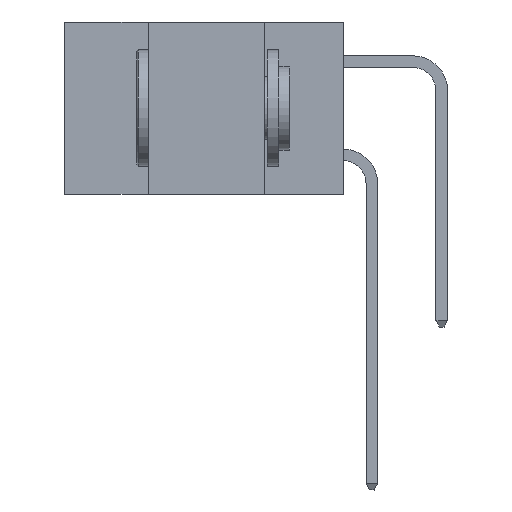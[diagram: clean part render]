
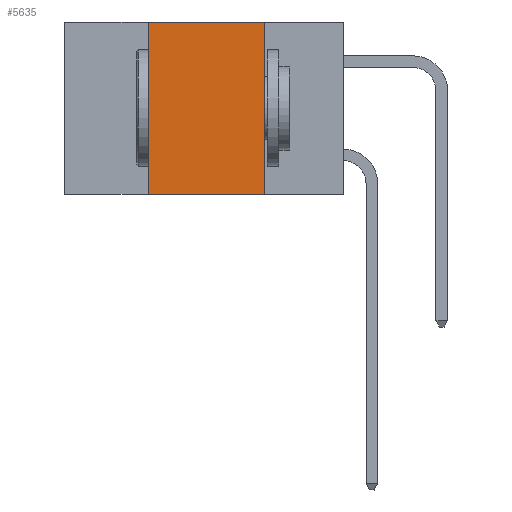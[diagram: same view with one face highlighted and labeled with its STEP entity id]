
A CAD part, left-side view. The second image highlights one B-rep face of the part: STEP entity #5635.
In plain terms, the highlighted planar face has unit normal (-1, 0, 0).
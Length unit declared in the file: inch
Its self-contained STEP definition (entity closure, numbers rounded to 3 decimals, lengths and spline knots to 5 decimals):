
#769 = CARTESIAN_POINT ( 'NONE',  ( 0., 0.17, 0. ) ) ;
#1058 = LINE ( 'NONE', #2823, #28242 ) ;
#1062 = EDGE_CURVE ( 'NONE', #29601, #11654, #19205, .T. ) ;
#1976 = CARTESIAN_POINT ( 'NONE',  ( 0., 0.6, -0.37 ) ) ;
#2430 = EDGE_LOOP ( 'NONE', ( #25160, #31575, #11569, #6998 ) ) ;
#2725 = CARTESIAN_POINT ( 'NONE',  ( 0., 0.6, 0. ) ) ;
#2823 = CARTESIAN_POINT ( 'NONE',  ( 0., 0.42, 0. ) ) ;
#3023 = CARTESIAN_POINT ( 'NONE',  ( 0., 0.6, 0. ) ) ;
#3676 = CARTESIAN_POINT ( 'NONE',  ( 0., 0.42, 0. ) ) ;
#4489 = VECTOR ( 'NONE', #7281, 39.37008 ) ;
#5635 = ADVANCED_FACE ( 'NONE', ( #14185 ), #13367, .F. ) ;
#6341 = EDGE_CURVE ( 'NONE', #23359, #29601, #26075, .T. ) ;
#6998 = ORIENTED_EDGE ( 'NONE', *, *, #12438, .T. ) ;
#7281 = DIRECTION ( 'NONE',  ( 0., -1., 0. ) ) ;
#7511 = VECTOR ( 'NONE', #29233, 39.37008 ) ;
#8779 = VERTEX_POINT ( 'NONE', #19629 ) ;
#11569 = ORIENTED_EDGE ( 'NONE', *, *, #28237, .F. ) ;
#11654 = VERTEX_POINT ( 'NONE', #12194 ) ;
#12194 = CARTESIAN_POINT ( 'NONE',  ( 0., 0.17, -0.37 ) ) ;
#12438 = EDGE_CURVE ( 'NONE', #8779, #11654, #31542, .T. ) ;
#13367 = PLANE ( 'NONE',  #28491 ) ;
#14185 = FACE_OUTER_BOUND ( 'NONE', #2430, .T. ) ;
#16051 = DIRECTION ( 'NONE',  ( 0., 0., -1. ) ) ;
#16392 = CARTESIAN_POINT ( 'NONE',  ( 0., 0.17, 0. ) ) ;
#17819 = DIRECTION ( 'NONE',  ( 0., 0., -1. ) ) ;
#19205 = LINE ( 'NONE', #769, #32135 ) ;
#19629 = CARTESIAN_POINT ( 'NONE',  ( 0., 0.42, -0.37 ) ) ;
#23359 = VERTEX_POINT ( 'NONE', #3676 ) ;
#25160 = ORIENTED_EDGE ( 'NONE', *, *, #1062, .F. ) ;
#26075 = LINE ( 'NONE', #3023, #7511 ) ;
#28237 = EDGE_CURVE ( 'NONE', #8779, #23359, #1058, .T. ) ;
#28242 = VECTOR ( 'NONE', #29035, 39.37008 ) ;
#28491 = AXIS2_PLACEMENT_3D ( 'NONE', #2725, #31625, #16051 ) ;
#29035 = DIRECTION ( 'NONE',  ( 0., 0., 1. ) ) ;
#29233 = DIRECTION ( 'NONE',  ( 0., -1., 0. ) ) ;
#29601 = VERTEX_POINT ( 'NONE', #16392 ) ;
#31542 = LINE ( 'NONE', #1976, #4489 ) ;
#31575 = ORIENTED_EDGE ( 'NONE', *, *, #6341, .F. ) ;
#31625 = DIRECTION ( 'NONE',  ( 1., 0., 0. ) ) ;
#32135 = VECTOR ( 'NONE', #17819, 39.37008 ) ;
